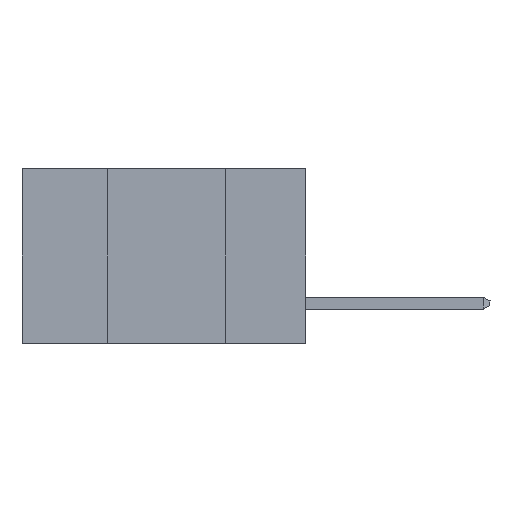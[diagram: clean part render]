
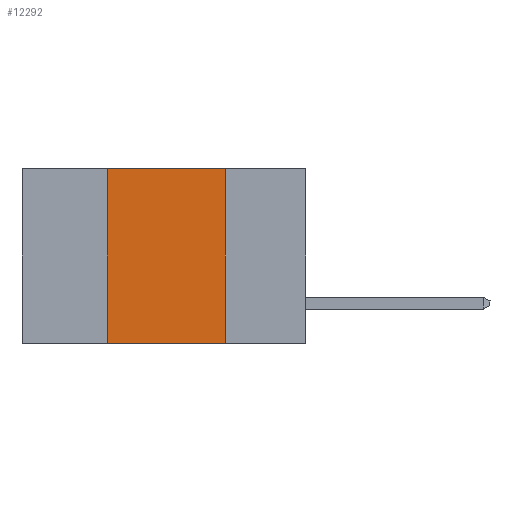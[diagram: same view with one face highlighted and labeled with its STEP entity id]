
A CAD part, left-side view. The second image highlights one B-rep face of the part: STEP entity #12292.
In plain terms, the highlighted planar face has unit normal (-1, 0, 0).
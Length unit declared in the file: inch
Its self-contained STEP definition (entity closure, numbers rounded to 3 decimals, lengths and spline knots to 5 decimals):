
#1080 = EDGE_CURVE ( 'NONE', #25254, #24030, #22387, .T. ) ;
#2311 = AXIS2_PLACEMENT_3D ( 'NONE', #27758, #25692, #4045 ) ;
#2878 = CARTESIAN_POINT ( 'NONE',  ( 0., 0.17, 0. ) ) ;
#3845 = LINE ( 'NONE', #12167, #18692 ) ;
#4045 = DIRECTION ( 'NONE',  ( 0., 0., -1. ) ) ;
#4088 = DIRECTION ( 'NONE',  ( 0., 0., -1. ) ) ;
#5494 = ORIENTED_EDGE ( 'NONE', *, *, #8039, .F. ) ;
#8039 = EDGE_CURVE ( 'NONE', #19529, #24030, #24064, .T. ) ;
#10175 = VECTOR ( 'NONE', #13675, 39.37008 ) ;
#11331 = LINE ( 'NONE', #16520, #18672 ) ;
#11473 = VECTOR ( 'NONE', #4088, 39.37008 ) ;
#12167 = CARTESIAN_POINT ( 'NONE',  ( 0., 0.42, 0. ) ) ;
#12292 = ADVANCED_FACE ( 'NONE', ( #15790 ), #20621, .F. ) ;
#12843 = ORIENTED_EDGE ( 'NONE', *, *, #1080, .T. ) ;
#13675 = DIRECTION ( 'NONE',  ( 0., -1., 0. ) ) ;
#15790 = FACE_OUTER_BOUND ( 'NONE', #25023, .T. ) ;
#16520 = CARTESIAN_POINT ( 'NONE',  ( 0., 0.6, 0. ) ) ;
#16990 = VERTEX_POINT ( 'NONE', #19917 ) ;
#18146 = CARTESIAN_POINT ( 'NONE',  ( 0., 0.42, -0.37 ) ) ;
#18672 = VECTOR ( 'NONE', #21071, 39.37008 ) ;
#18692 = VECTOR ( 'NONE', #28753, 39.37008 ) ;
#19529 = VERTEX_POINT ( 'NONE', #22028 ) ;
#19917 = CARTESIAN_POINT ( 'NONE',  ( 0., 0.42, 0. ) ) ;
#20621 = PLANE ( 'NONE',  #2311 ) ;
#20718 = CARTESIAN_POINT ( 'NONE',  ( 0., 0.6, -0.37 ) ) ;
#21071 = DIRECTION ( 'NONE',  ( 0., -1., 0. ) ) ;
#22028 = CARTESIAN_POINT ( 'NONE',  ( 0., 0.17, 0. ) ) ;
#22141 = CARTESIAN_POINT ( 'NONE',  ( 0., 0.17, -0.37 ) ) ;
#22387 = LINE ( 'NONE', #20718, #10175 ) ;
#23346 = ORIENTED_EDGE ( 'NONE', *, *, #30116, .F. ) ;
#24030 = VERTEX_POINT ( 'NONE', #22141 ) ;
#24064 = LINE ( 'NONE', #2878, #11473 ) ;
#24319 = EDGE_CURVE ( 'NONE', #16990, #19529, #11331, .T. ) ;
#25023 = EDGE_LOOP ( 'NONE', ( #5494, #28556, #23346, #12843 ) ) ;
#25254 = VERTEX_POINT ( 'NONE', #18146 ) ;
#25692 = DIRECTION ( 'NONE',  ( 1., 0., 0. ) ) ;
#27758 = CARTESIAN_POINT ( 'NONE',  ( 0., 0.6, 0. ) ) ;
#28556 = ORIENTED_EDGE ( 'NONE', *, *, #24319, .F. ) ;
#28753 = DIRECTION ( 'NONE',  ( 0., 0., 1. ) ) ;
#30116 = EDGE_CURVE ( 'NONE', #25254, #16990, #3845, .T. ) ;
